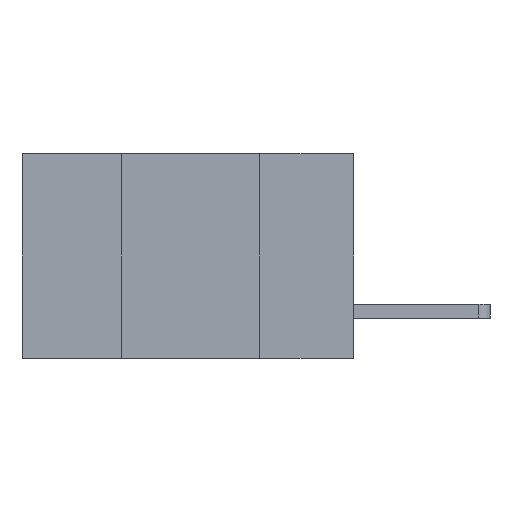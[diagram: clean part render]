
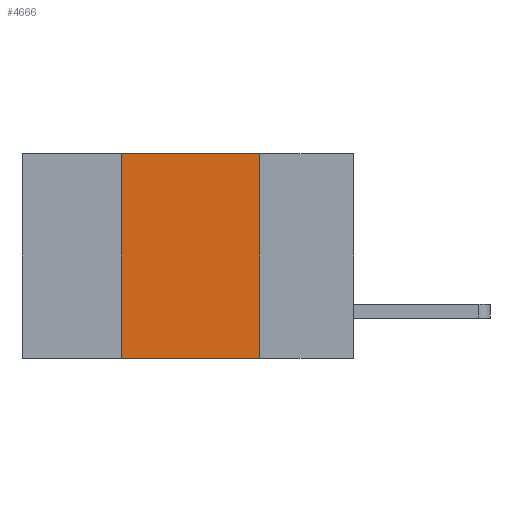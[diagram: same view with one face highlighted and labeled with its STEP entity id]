
A CAD part, left-side view. The second image highlights one B-rep face of the part: STEP entity #4666.
In plain terms, the highlighted planar face has unit normal (-1, 0, 0).
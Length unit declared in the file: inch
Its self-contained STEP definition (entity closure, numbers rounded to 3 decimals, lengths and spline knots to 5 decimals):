
#243 = VECTOR ( 'NONE', #5174, 39.37008 ) ;
#305 = VERTEX_POINT ( 'NONE', #5841 ) ;
#605 = VERTEX_POINT ( 'NONE', #8977 ) ;
#619 = ORIENTED_EDGE ( 'NONE', *, *, #3463, .T. ) ;
#987 = ORIENTED_EDGE ( 'NONE', *, *, #2528, .F. ) ;
#1065 = ORIENTED_EDGE ( 'NONE', *, *, #3659, .F. ) ;
#1281 = ORIENTED_EDGE ( 'NONE', *, *, #3303, .F. ) ;
#1545 = LINE ( 'NONE', #7337, #7803 ) ;
#2496 = VECTOR ( 'NONE', #10310, 39.37008 ) ;
#2528 = EDGE_CURVE ( 'NONE', #5504, #3720, #7043, .T. ) ;
#3303 = EDGE_CURVE ( 'NONE', #305, #605, #1545, .T. ) ;
#3429 = AXIS2_PLACEMENT_3D ( 'NONE', #8200, #5368, #4455 ) ;
#3463 = EDGE_CURVE ( 'NONE', #305, #3720, #6764, .T. ) ;
#3659 = EDGE_CURVE ( 'NONE', #605, #5504, #4850, .T. ) ;
#3678 = EDGE_LOOP ( 'NONE', ( #987, #1065, #1281, #619 ) ) ;
#3720 = VERTEX_POINT ( 'NONE', #5060 ) ;
#4455 = DIRECTION ( 'NONE',  ( 0., 0., -1. ) ) ;
#4666 = ADVANCED_FACE ( 'NONE', ( #9559 ), #4893, .F. ) ;
#4850 = LINE ( 'NONE', #5063, #243 ) ;
#4893 = PLANE ( 'NONE',  #3429 ) ;
#4923 = DIRECTION ( 'NONE',  ( 0., -1., 0. ) ) ;
#5060 = CARTESIAN_POINT ( 'NONE',  ( 0., 0.17, -0.37 ) ) ;
#5063 = CARTESIAN_POINT ( 'NONE',  ( 0., 0.6, 0. ) ) ;
#5137 = CARTESIAN_POINT ( 'NONE',  ( 0., 0.17, 0. ) ) ;
#5174 = DIRECTION ( 'NONE',  ( 0., -1., 0. ) ) ;
#5368 = DIRECTION ( 'NONE',  ( 1., 0., 0. ) ) ;
#5504 = VERTEX_POINT ( 'NONE', #5137 ) ;
#5533 = CARTESIAN_POINT ( 'NONE',  ( 0., 0.17, 0. ) ) ;
#5841 = CARTESIAN_POINT ( 'NONE',  ( 0., 0.42, -0.37 ) ) ;
#6519 = VECTOR ( 'NONE', #4923, 39.37008 ) ;
#6764 = LINE ( 'NONE', #6971, #6519 ) ;
#6971 = CARTESIAN_POINT ( 'NONE',  ( 0., 0.6, -0.37 ) ) ;
#7043 = LINE ( 'NONE', #5533, #2496 ) ;
#7337 = CARTESIAN_POINT ( 'NONE',  ( 0., 0.42, 0. ) ) ;
#7627 = DIRECTION ( 'NONE',  ( 0., 0., 1. ) ) ;
#7803 = VECTOR ( 'NONE', #7627, 39.37008 ) ;
#8200 = CARTESIAN_POINT ( 'NONE',  ( 0., 0.6, 0. ) ) ;
#8977 = CARTESIAN_POINT ( 'NONE',  ( 0., 0.42, 0. ) ) ;
#9559 = FACE_OUTER_BOUND ( 'NONE', #3678, .T. ) ;
#10310 = DIRECTION ( 'NONE',  ( 0., 0., -1. ) ) ;
